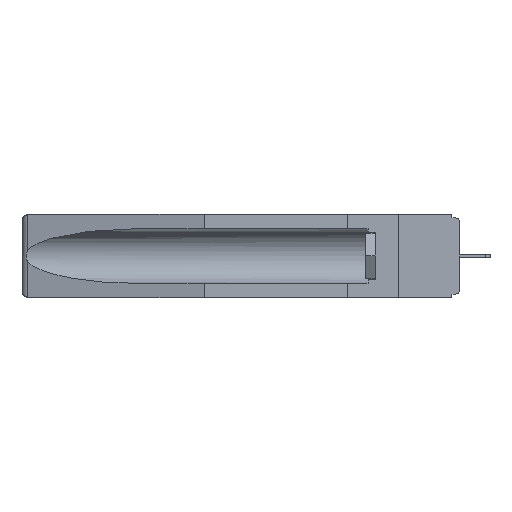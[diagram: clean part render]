
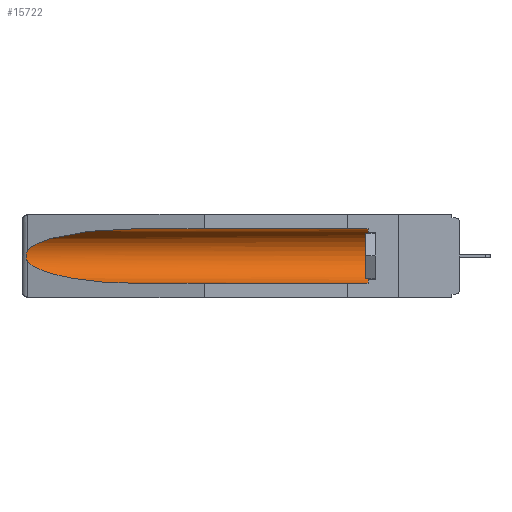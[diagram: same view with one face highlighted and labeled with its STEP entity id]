
A CAD part, left-side view. The second image highlights one B-rep face of the part: STEP entity #15722.
In plain terms, the highlighted cylindrical face has radius 2.857 mm (diameter 5.715 mm), a partial arc.
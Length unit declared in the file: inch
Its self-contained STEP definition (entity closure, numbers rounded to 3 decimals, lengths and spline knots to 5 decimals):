
#175 = CARTESIAN_POINT ( 'NONE',  ( 0.26537, 1.52718, -0.19328 ) ) ;
#349 = CARTESIAN_POINT ( 'NONE',  ( 0.155, 1.07973, -0.284 ) ) ;
#679 = CIRCLE ( 'NONE', #14636, 0.1125 ) ;
#856 = EDGE_CURVE ( 'NONE', #14176, #7369, #11075, .T. ) ;
#992 = DIRECTION ( 'NONE',  ( 0., 1., 0. ) ) ;
#1764 =( BOUNDED_CURVE ( )  B_SPLINE_CURVE ( 3, ( #17256, #18812, #9342, #20379 ),
 .UNSPECIFIED., .F., .F. ) 
 B_SPLINE_CURVE_WITH_KNOTS ( ( 4, 4 ),
 ( 4.71239, 6.08839 ),
 .UNSPECIFIED. ) 
 CURVE ( )  GEOMETRIC_REPRESENTATION_ITEM ( )  RATIONAL_B_SPLINE_CURVE ( ( 1., 0.848, 0.848, 1. ) ) 
 REPRESENTATION_ITEM ( '' )  );
#2534 = CARTESIAN_POINT ( 'NONE',  ( 0.26537, 1.52718, -0.14972 ) ) ;
#2977 = CYLINDRICAL_SURFACE ( 'NONE', #6926, 0.1125 ) ;
#3190 = EDGE_CURVE ( 'NONE', #15223, #3600, #8715, .T. ) ;
#3405 = VERTEX_POINT ( 'NONE', #175 ) ;
#3436 = EDGE_CURVE ( 'NONE', #6934, #3405, #7117, .T. ) ;
#3546 = DIRECTION ( 'NONE',  ( 0., 1., 0. ) ) ;
#3558 = CARTESIAN_POINT ( 'NONE',  ( 0.155, 0.126, -0.059 ) ) ;
#3600 = VERTEX_POINT ( 'NONE', #9339 ) ;
#4756 = CARTESIAN_POINT ( 'NONE',  ( 0.155, -0.30754, -0.1715 ) ) ;
#5399 = CARTESIAN_POINT ( 'NONE',  ( 0.2673, 1.53269, -0.17917 ) ) ;
#5541 =( BOUNDED_CURVE ( )  B_SPLINE_CURVE ( 3, ( #10571, #5779, #9045, #20101 ),
 .UNSPECIFIED., .F., .F. ) 
 B_SPLINE_CURVE_WITH_KNOTS ( ( 4, 4 ),
 ( 0.1948, 1.5708 ),
 .UNSPECIFIED. ) 
 CURVE ( )  GEOMETRIC_REPRESENTATION_ITEM ( )  RATIONAL_B_SPLINE_CURVE ( ( 1., 0.848, 0.848, 1. ) ) 
 REPRESENTATION_ITEM ( '' )  );
#5779 = CARTESIAN_POINT ( 'NONE',  ( 0.25451, 1.48313, -0.24835 ) ) ;
#6047 = CARTESIAN_POINT ( 'NONE',  ( 0.155, -0.30754, -0.059 ) ) ;
#6400 = DIRECTION ( 'NONE',  ( 0., 0., 1. ) ) ;
#6926 = AXIS2_PLACEMENT_3D ( 'NONE', #4756, #9643, #6400 ) ;
#6934 = VERTEX_POINT ( 'NONE', #2534 ) ;
#7117 = B_SPLINE_CURVE_WITH_KNOTS ( 'NONE', 3,
 ( #14190, #17250, #15892, #18177, #8686, #15032, #5399, #16616, #19352, #18417 ),
 .UNSPECIFIED., .F., .F.,
 ( 4, 2, 2, 2, 4 ),
 ( 0., 0.00029, 0.00058, 0.00087, 0.00117 ),
 .UNSPECIFIED. ) ;
#7239 = ORIENTED_EDGE ( 'NONE', *, *, #10893, .T. ) ;
#7369 = VERTEX_POINT ( 'NONE', #349 ) ;
#8346 = FACE_OUTER_BOUND ( 'NONE', #9128, .T. ) ;
#8634 = DIRECTION ( 'NONE',  ( 0., -1., 0. ) ) ;
#8686 = CARTESIAN_POINT ( 'NONE',  ( 0.2675, 1.53308, -0.16763 ) ) ;
#8715 = LINE ( 'NONE', #6047, #16676 ) ;
#8735 = CARTESIAN_POINT ( 'NONE',  ( 0.155, 0.126, -0.284 ) ) ;
#9045 = CARTESIAN_POINT ( 'NONE',  ( 0.21114, 1.30732, -0.284 ) ) ;
#9128 = EDGE_LOOP ( 'NONE', ( #11597, #9508, #7239, #18546, #18793, #16152 ) ) ;
#9339 = CARTESIAN_POINT ( 'NONE',  ( 0.155, 1.07973, -0.059 ) ) ;
#9342 = CARTESIAN_POINT ( 'NONE',  ( 0.25451, 1.48313, -0.09465 ) ) ;
#9508 = ORIENTED_EDGE ( 'NONE', *, *, #3436, .T. ) ;
#9643 = DIRECTION ( 'NONE',  ( 0., 1., 0. ) ) ;
#10571 = CARTESIAN_POINT ( 'NONE',  ( 0.26537, 1.52718, -0.19328 ) ) ;
#10893 = EDGE_CURVE ( 'NONE', #3405, #7369, #5541, .T. ) ;
#10952 = EDGE_CURVE ( 'NONE', #3600, #6934, #1764, .T. ) ;
#11075 = LINE ( 'NONE', #17582, #18975 ) ;
#11597 = ORIENTED_EDGE ( 'NONE', *, *, #10952, .T. ) ;
#11809 = EDGE_CURVE ( 'NONE', #14176, #15223, #679, .T. ) ;
#14176 = VERTEX_POINT ( 'NONE', #8735 ) ;
#14190 = CARTESIAN_POINT ( 'NONE',  ( 0.26537, 1.52718, -0.14972 ) ) ;
#14636 = AXIS2_PLACEMENT_3D ( 'NONE', #18120, #8634, #19690 ) ;
#15032 = CARTESIAN_POINT ( 'NONE',  ( 0.2675, 1.53308, -0.17534 ) ) ;
#15223 = VERTEX_POINT ( 'NONE', #3558 ) ;
#15722 = ADVANCED_FACE ( 'NONE', ( #8346 ), #2977, .F. ) ;
#15892 = CARTESIAN_POINT ( 'NONE',  ( 0.26654, 1.53092, -0.15636 ) ) ;
#16152 = ORIENTED_EDGE ( 'NONE', *, *, #3190, .T. ) ;
#16616 = CARTESIAN_POINT ( 'NONE',  ( 0.26655, 1.53094, -0.18657 ) ) ;
#16676 = VECTOR ( 'NONE', #3546, 39.37008 ) ;
#17250 = CARTESIAN_POINT ( 'NONE',  ( 0.26597, 1.52961, -0.15275 ) ) ;
#17256 = CARTESIAN_POINT ( 'NONE',  ( 0.155, 1.07973, -0.059 ) ) ;
#17582 = CARTESIAN_POINT ( 'NONE',  ( 0.155, -0.30754, -0.284 ) ) ;
#18120 = CARTESIAN_POINT ( 'NONE',  ( 0.155, 0.126, -0.1715 ) ) ;
#18177 = CARTESIAN_POINT ( 'NONE',  ( 0.2673, 1.5327, -0.16383 ) ) ;
#18417 = CARTESIAN_POINT ( 'NONE',  ( 0.26537, 1.52718, -0.19328 ) ) ;
#18546 = ORIENTED_EDGE ( 'NONE', *, *, #856, .F. ) ;
#18793 = ORIENTED_EDGE ( 'NONE', *, *, #11809, .T. ) ;
#18812 = CARTESIAN_POINT ( 'NONE',  ( 0.21114, 1.30732, -0.059 ) ) ;
#18975 = VECTOR ( 'NONE', #992, 39.37008 ) ;
#19352 = CARTESIAN_POINT ( 'NONE',  ( 0.26597, 1.5296, -0.19026 ) ) ;
#19690 = DIRECTION ( 'NONE',  ( 0., 0., 1. ) ) ;
#20101 = CARTESIAN_POINT ( 'NONE',  ( 0.155, 1.07973, -0.284 ) ) ;
#20379 = CARTESIAN_POINT ( 'NONE',  ( 0.26537, 1.52718, -0.14972 ) ) ;
